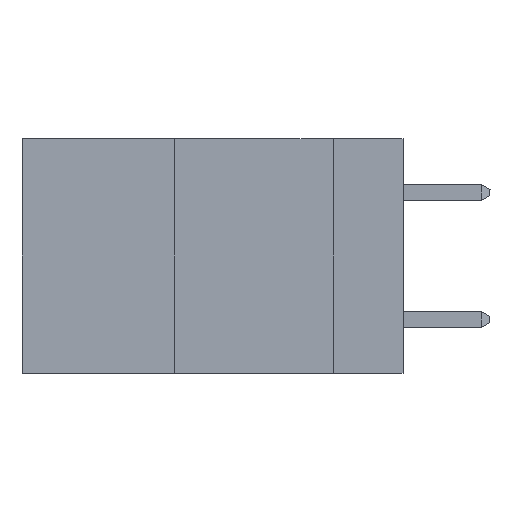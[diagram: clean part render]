
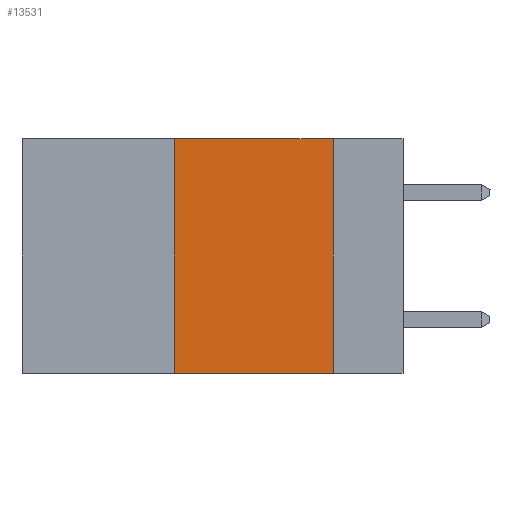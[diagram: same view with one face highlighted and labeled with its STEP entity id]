
A CAD part, left-side view. The second image highlights one B-rep face of the part: STEP entity #13531.
In plain terms, the highlighted planar face has unit normal (-1, 0, 0).
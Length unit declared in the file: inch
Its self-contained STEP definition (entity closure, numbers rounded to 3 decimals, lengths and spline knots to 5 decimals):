
#218 = VERTEX_POINT ( 'NONE', #8212 ) ;
#281 = CARTESIAN_POINT ( 'NONE',  ( 0., 0.11, -0.37 ) ) ;
#1657 = EDGE_LOOP ( 'NONE', ( #10078, #13265, #2121, #11432 ) ) ;
#1883 = FACE_OUTER_BOUND ( 'NONE', #1657, .T. ) ;
#2121 = ORIENTED_EDGE ( 'NONE', *, *, #14042, .F. ) ;
#2155 = CARTESIAN_POINT ( 'NONE',  ( 0., 0.11, 0. ) ) ;
#2725 = VECTOR ( 'NONE', #4948, 39.37008 ) ;
#3200 = LINE ( 'NONE', #6528, #11974 ) ;
#3467 = PLANE ( 'NONE',  #13125 ) ;
#3975 = DIRECTION ( 'NONE',  ( 0., -1., 0. ) ) ;
#4428 = CARTESIAN_POINT ( 'NONE',  ( 0., 0.6, 0. ) ) ;
#4553 = LINE ( 'NONE', #5230, #10921 ) ;
#4689 = LINE ( 'NONE', #4428, #13642 ) ;
#4777 = DIRECTION ( 'NONE',  ( 1., 0., 0. ) ) ;
#4948 = DIRECTION ( 'NONE',  ( 0., 0., 1. ) ) ;
#5230 = CARTESIAN_POINT ( 'NONE',  ( 0., 0.6, -0.37 ) ) ;
#5641 = LINE ( 'NONE', #10436, #2725 ) ;
#5712 = EDGE_CURVE ( 'NONE', #6183, #5933, #3200, .T. ) ;
#5933 = VERTEX_POINT ( 'NONE', #281 ) ;
#6183 = VERTEX_POINT ( 'NONE', #2155 ) ;
#6528 = CARTESIAN_POINT ( 'NONE',  ( 0., 0.11, 0. ) ) ;
#8212 = CARTESIAN_POINT ( 'NONE',  ( 0., 0.36, 0. ) ) ;
#8557 = CARTESIAN_POINT ( 'NONE',  ( 0., 0.36, -0.37 ) ) ;
#9300 = DIRECTION ( 'NONE',  ( 0., 0., -1. ) ) ;
#9491 = EDGE_CURVE ( 'NONE', #9540, #5933, #4553, .T. ) ;
#9540 = VERTEX_POINT ( 'NONE', #8557 ) ;
#10078 = ORIENTED_EDGE ( 'NONE', *, *, #5712, .F. ) ;
#10436 = CARTESIAN_POINT ( 'NONE',  ( 0., 0.36, 0. ) ) ;
#10869 = EDGE_CURVE ( 'NONE', #218, #6183, #4689, .T. ) ;
#10921 = VECTOR ( 'NONE', #3975, 39.37008 ) ;
#11378 = CARTESIAN_POINT ( 'NONE',  ( 0., 0.6, 0. ) ) ;
#11432 = ORIENTED_EDGE ( 'NONE', *, *, #9491, .T. ) ;
#11974 = VECTOR ( 'NONE', #14227, 39.37008 ) ;
#12406 = DIRECTION ( 'NONE',  ( 0., -1., 0. ) ) ;
#13125 = AXIS2_PLACEMENT_3D ( 'NONE', #11378, #4777, #9300 ) ;
#13265 = ORIENTED_EDGE ( 'NONE', *, *, #10869, .F. ) ;
#13531 = ADVANCED_FACE ( 'NONE', ( #1883 ), #3467, .F. ) ;
#13642 = VECTOR ( 'NONE', #12406, 39.37008 ) ;
#14042 = EDGE_CURVE ( 'NONE', #9540, #218, #5641, .T. ) ;
#14227 = DIRECTION ( 'NONE',  ( 0., 0., -1. ) ) ;
